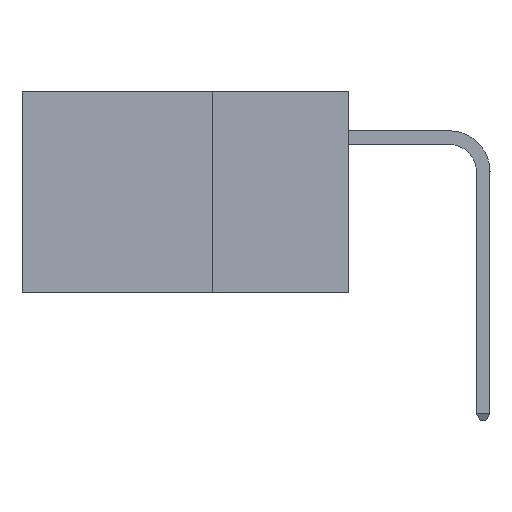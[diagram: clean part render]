
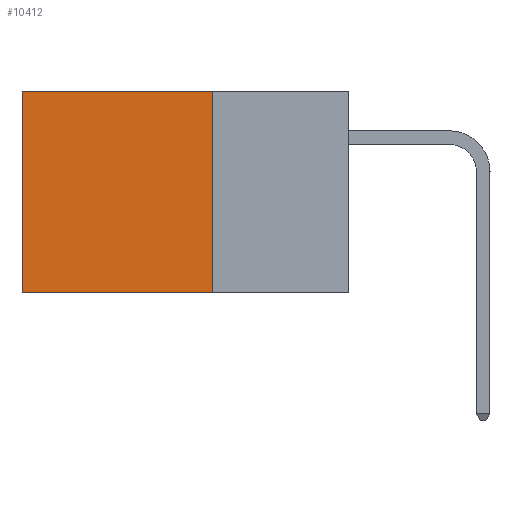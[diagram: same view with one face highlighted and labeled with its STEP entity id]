
A CAD part, left-side view. The second image highlights one B-rep face of the part: STEP entity #10412.
In plain terms, the highlighted planar face has unit normal (-1, 0, 0).
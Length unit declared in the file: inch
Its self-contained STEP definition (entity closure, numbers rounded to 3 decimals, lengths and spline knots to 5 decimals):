
#131 = VECTOR ( 'NONE', #7058, 39.37008 ) ;
#676 = LINE ( 'NONE', #4856, #131 ) ;
#980 = CARTESIAN_POINT ( 'NONE',  ( 0.2875, 0.25, 0. ) ) ;
#1880 = PLANE ( 'NONE',  #9097 ) ;
#2116 = DIRECTION ( 'NONE',  ( 0., 1., 0. ) ) ;
#2514 = EDGE_CURVE ( 'NONE', #7662, #9542, #2537, .T. ) ;
#2537 = LINE ( 'NONE', #4793, #9645 ) ;
#2702 = CARTESIAN_POINT ( 'NONE',  ( 0.2875, 0.25, -0.37 ) ) ;
#3204 = CARTESIAN_POINT ( 'NONE',  ( 0.2875, 0.25, 0. ) ) ;
#3405 = VERTEX_POINT ( 'NONE', #7593 ) ;
#3497 = DIRECTION ( 'NONE',  ( 0., 0., -1. ) ) ;
#3716 = CARTESIAN_POINT ( 'NONE',  ( 0.2875, 0.25, -0.37 ) ) ;
#3932 = VECTOR ( 'NONE', #2116, 39.37008 ) ;
#3998 = DIRECTION ( 'NONE',  ( 0., 0., -1. ) ) ;
#4270 = VECTOR ( 'NONE', #11144, 39.37008 ) ;
#4793 = CARTESIAN_POINT ( 'NONE',  ( 0.2875, 0.25, 0. ) ) ;
#4856 = CARTESIAN_POINT ( 'NONE',  ( 0.2875, 0.6, 0. ) ) ;
#6453 = ORIENTED_EDGE ( 'NONE', *, *, #2514, .F. ) ;
#6466 = EDGE_CURVE ( 'NONE', #9542, #3405, #8950, .T. ) ;
#7058 = DIRECTION ( 'NONE',  ( 0., 0., -1. ) ) ;
#7228 = DIRECTION ( 'NONE',  ( 1., 0., 0. ) ) ;
#7339 = EDGE_CURVE ( 'NONE', #8665, #3405, #676, .T. ) ;
#7593 = CARTESIAN_POINT ( 'NONE',  ( 0.2875, 0.6, -0.37 ) ) ;
#7662 = VERTEX_POINT ( 'NONE', #10957 ) ;
#8433 = LINE ( 'NONE', #3204, #3932 ) ;
#8665 = VERTEX_POINT ( 'NONE', #10159 ) ;
#8950 = LINE ( 'NONE', #3716, #4270 ) ;
#8994 = EDGE_LOOP ( 'NONE', ( #10402, #13243, #6453, #9371 ) ) ;
#9097 = AXIS2_PLACEMENT_3D ( 'NONE', #980, #7228, #3998 ) ;
#9371 = ORIENTED_EDGE ( 'NONE', *, *, #12528, .T. ) ;
#9542 = VERTEX_POINT ( 'NONE', #2702 ) ;
#9645 = VECTOR ( 'NONE', #3497, 39.37008 ) ;
#10159 = CARTESIAN_POINT ( 'NONE',  ( 0.2875, 0.6, 0. ) ) ;
#10402 = ORIENTED_EDGE ( 'NONE', *, *, #7339, .T. ) ;
#10412 = ADVANCED_FACE ( 'NONE', ( #11289 ), #1880, .F. ) ;
#10957 = CARTESIAN_POINT ( 'NONE',  ( 0.2875, 0.25, 0. ) ) ;
#11144 = DIRECTION ( 'NONE',  ( 0., 1., 0. ) ) ;
#11289 = FACE_OUTER_BOUND ( 'NONE', #8994, .T. ) ;
#12528 = EDGE_CURVE ( 'NONE', #7662, #8665, #8433, .T. ) ;
#13243 = ORIENTED_EDGE ( 'NONE', *, *, #6466, .F. ) ;
